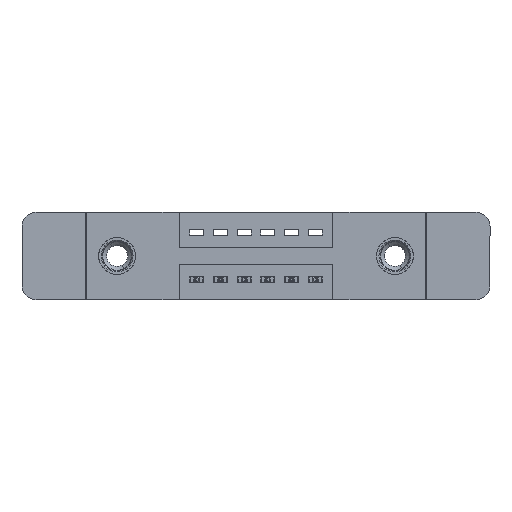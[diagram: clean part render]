
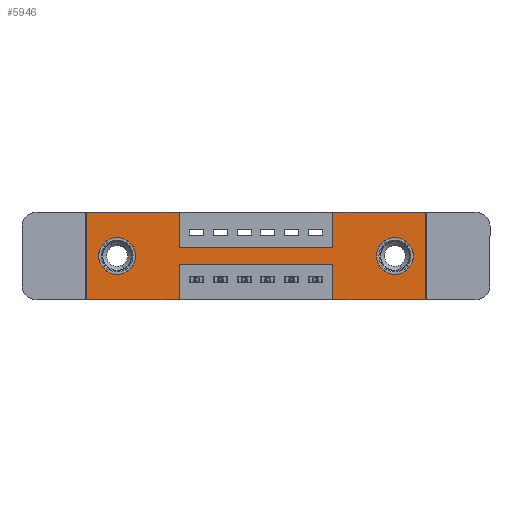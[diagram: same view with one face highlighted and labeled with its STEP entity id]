
A CAD part, front view. The second image highlights one B-rep face of the part: STEP entity #5946.
In plain terms, the highlighted planar face has unit normal (0, -1, 0).
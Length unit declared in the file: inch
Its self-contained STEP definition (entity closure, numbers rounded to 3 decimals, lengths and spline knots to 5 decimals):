
#244 = LINE ( 'NONE', #13794, #6252 ) ;
#265 = CIRCLE ( 'NONE', #1947, 0.078 ) ;
#278 = DIRECTION ( 'NONE',  ( 0., 0., -1. ) ) ;
#378 = DIRECTION ( 'NONE',  ( 0., 0., 1. ) ) ;
#475 = DIRECTION ( 'NONE',  ( -1., 0., 0. ) ) ;
#531 = VERTEX_POINT ( 'NONE', #13486 ) ;
#538 = VECTOR ( 'NONE', #7773, 39.37008 ) ;
#620 = CARTESIAN_POINT ( 'NONE',  ( 1.435, 0., -0.37 ) ) ;
#1287 = CIRCLE ( 'NONE', #2014, 0.078 ) ;
#1378 = EDGE_CURVE ( 'NONE', #5949, #7877, #12504, .T. ) ;
#1595 = VERTEX_POINT ( 'NONE', #13214 ) ;
#1741 = VECTOR ( 'NONE', #378, 39.37008 ) ;
#1817 = CARTESIAN_POINT ( 'NONE',  ( 0.3925, 0., -0.37 ) ) ;
#1819 = CARTESIAN_POINT ( 'NONE',  ( 0.3925, 0., -0.22 ) ) ;
#1947 = AXIS2_PLACEMENT_3D ( 'NONE', #5736, #12311, #6732 ) ;
#2014 = AXIS2_PLACEMENT_3D ( 'NONE', #12330, #12384, #6898 ) ;
#2072 = FACE_OUTER_BOUND ( 'NONE', #3925, .T. ) ;
#2209 = LINE ( 'NONE', #10895, #4870 ) ;
#2354 = VECTOR ( 'NONE', #8885, 39.37008 ) ;
#2723 = CARTESIAN_POINT ( 'NONE',  ( 1.0425, 0., 0. ) ) ;
#3039 = LINE ( 'NONE', #3862, #11682 ) ;
#3055 = CARTESIAN_POINT ( 'NONE',  ( 1.435, 0., 0. ) ) ;
#3166 = DIRECTION ( 'NONE',  ( 0., 0., -1. ) ) ;
#3187 = ORIENTED_EDGE ( 'NONE', *, *, #11785, .F. ) ;
#3298 = ORIENTED_EDGE ( 'NONE', *, *, #3936, .T. ) ;
#3303 = EDGE_CURVE ( 'NONE', #11059, #5215, #2209, .T. ) ;
#3304 = CARTESIAN_POINT ( 'NONE',  ( 1.0425, 0., -0.37 ) ) ;
#3393 = EDGE_CURVE ( 'NONE', #8481, #11059, #3789, .T. ) ;
#3515 = ORIENTED_EDGE ( 'NONE', *, *, #5880, .F. ) ;
#3595 = ORIENTED_EDGE ( 'NONE', *, *, #4989, .F. ) ;
#3655 = LINE ( 'NONE', #1819, #14251 ) ;
#3694 = DIRECTION ( 'NONE',  ( 0., 0., 1. ) ) ;
#3729 = LINE ( 'NONE', #3304, #538 ) ;
#3732 = CARTESIAN_POINT ( 'NONE',  ( 0., 0., 0. ) ) ;
#3789 = LINE ( 'NONE', #10486, #4155 ) ;
#3862 = CARTESIAN_POINT ( 'NONE',  ( 0., 0., 0. ) ) ;
#3925 = EDGE_LOOP ( 'NONE', ( #3595, #3515, #12734, #8670, #6734, #3187, #5157, #13919, #9355, #14100, #12618, #5961 ) ) ;
#3936 = EDGE_CURVE ( 'NONE', #531, #1595, #1287, .T. ) ;
#4110 = CARTESIAN_POINT ( 'NONE',  ( 1.0425, 0., -0.37 ) ) ;
#4155 = VECTOR ( 'NONE', #278, 39.37008 ) ;
#4364 = FACE_BOUND ( 'NONE', #7236, .T. ) ;
#4395 = CARTESIAN_POINT ( 'NONE',  ( 0., 0., -0.37 ) ) ;
#4492 = VECTOR ( 'NONE', #12124, 39.37008 ) ;
#4704 = EDGE_CURVE ( 'NONE', #14498, #14072, #244, .T. ) ;
#4748 = LINE ( 'NONE', #3732, #1741 ) ;
#4870 = VECTOR ( 'NONE', #12179, 39.37008 ) ;
#4989 = EDGE_CURVE ( 'NONE', #8682, #8084, #9417, .T. ) ;
#5077 = FACE_BOUND ( 'NONE', #5146, .T. ) ;
#5146 = EDGE_LOOP ( 'NONE', ( #13066, #9958 ) ) ;
#5157 = ORIENTED_EDGE ( 'NONE', *, *, #9910, .F. ) ;
#5215 = VERTEX_POINT ( 'NONE', #8140 ) ;
#5351 = CARTESIAN_POINT ( 'NONE',  ( 0.3925, 0., -0.37 ) ) ;
#5736 = CARTESIAN_POINT ( 'NONE',  ( 1.305, 0., -0.185 ) ) ;
#5878 = CARTESIAN_POINT ( 'NONE',  ( 1.0425, 0., 0. ) ) ;
#5880 = EDGE_CURVE ( 'NONE', #12254, #8682, #3655, .T. ) ;
#5946 = ADVANCED_FACE ( 'NONE', ( #5077, #4364, #2072 ), #7278, .T. ) ;
#5949 = VERTEX_POINT ( 'NONE', #8812 ) ;
#5961 = ORIENTED_EDGE ( 'NONE', *, *, #9845, .F. ) ;
#6208 = VECTOR ( 'NONE', #8326, 39.37008 ) ;
#6252 = VECTOR ( 'NONE', #8192, 39.37008 ) ;
#6527 = CARTESIAN_POINT ( 'NONE',  ( 1.0425, 0., -0.22 ) ) ;
#6732 = DIRECTION ( 'NONE',  ( 0., 0., -1. ) ) ;
#6734 = ORIENTED_EDGE ( 'NONE', *, *, #7230, .F. ) ;
#6753 = VERTEX_POINT ( 'NONE', #14349 ) ;
#6898 = DIRECTION ( 'NONE',  ( 0., 0., 1. ) ) ;
#6901 = EDGE_CURVE ( 'NONE', #7877, #5949, #265, .T. ) ;
#7230 = EDGE_CURVE ( 'NONE', #6753, #14498, #11904, .T. ) ;
#7236 = EDGE_LOOP ( 'NONE', ( #3298, #9581 ) ) ;
#7278 = PLANE ( 'NONE',  #9398 ) ;
#7397 = DIRECTION ( 'NONE',  ( 0., 1., 0. ) ) ;
#7773 = DIRECTION ( 'NONE',  ( 0., 0., 1. ) ) ;
#7777 = LINE ( 'NONE', #9518, #6208 ) ;
#7877 = VERTEX_POINT ( 'NONE', #10804 ) ;
#8084 = VERTEX_POINT ( 'NONE', #1817 ) ;
#8132 = VECTOR ( 'NONE', #10605, 39.37008 ) ;
#8140 = CARTESIAN_POINT ( 'NONE',  ( 1.0425, 0., -0.15 ) ) ;
#8192 = DIRECTION ( 'NONE',  ( -1., 0., 0. ) ) ;
#8256 = LINE ( 'NONE', #12017, #10922 ) ;
#8326 = DIRECTION ( 'NONE',  ( -1., 0., 0. ) ) ;
#8481 = VERTEX_POINT ( 'NONE', #8691 ) ;
#8543 = VERTEX_POINT ( 'NONE', #9862 ) ;
#8610 = CARTESIAN_POINT ( 'NONE',  ( 0., 0., -0.37 ) ) ;
#8663 = DIRECTION ( 'NONE',  ( 0., 0., -1. ) ) ;
#8670 = ORIENTED_EDGE ( 'NONE', *, *, #4704, .F. ) ;
#8682 = VERTEX_POINT ( 'NONE', #10302 ) ;
#8691 = CARTESIAN_POINT ( 'NONE',  ( 0.3925, 0., 0. ) ) ;
#8812 = CARTESIAN_POINT ( 'NONE',  ( 1.305, 0., -0.263 ) ) ;
#8885 = DIRECTION ( 'NONE',  ( 0., 0., -1. ) ) ;
#9355 = ORIENTED_EDGE ( 'NONE', *, *, #3393, .F. ) ;
#9398 = AXIS2_PLACEMENT_3D ( 'NONE', #8610, #12112, #8663 ) ;
#9417 = LINE ( 'NONE', #5351, #2354 ) ;
#9518 = CARTESIAN_POINT ( 'NONE',  ( 0., 0., -0.37 ) ) ;
#9581 = ORIENTED_EDGE ( 'NONE', *, *, #14347, .T. ) ;
#9617 = VERTEX_POINT ( 'NONE', #5878 ) ;
#9845 = EDGE_CURVE ( 'NONE', #8084, #11136, #7777, .T. ) ;
#9862 = CARTESIAN_POINT ( 'NONE',  ( 0., 0., 0. ) ) ;
#9910 = EDGE_CURVE ( 'NONE', #5215, #9617, #13995, .T. ) ;
#9947 = EDGE_CURVE ( 'NONE', #8543, #8481, #3039, .T. ) ;
#9958 = ORIENTED_EDGE ( 'NONE', *, *, #1378, .T. ) ;
#10144 = EDGE_CURVE ( 'NONE', #14072, #12254, #3729, .T. ) ;
#10236 = DIRECTION ( 'NONE',  ( 0., 1., 0. ) ) ;
#10285 = CARTESIAN_POINT ( 'NONE',  ( 0.13, 0., -0.185 ) ) ;
#10302 = CARTESIAN_POINT ( 'NONE',  ( 0.3925, 0., -0.22 ) ) ;
#10486 = CARTESIAN_POINT ( 'NONE',  ( 0.3925, 0., 0. ) ) ;
#10605 = DIRECTION ( 'NONE',  ( 0., 0., 1. ) ) ;
#10804 = CARTESIAN_POINT ( 'NONE',  ( 1.305, 0., -0.107 ) ) ;
#10861 = CARTESIAN_POINT ( 'NONE',  ( 0.3925, 0., -0.15 ) ) ;
#10895 = CARTESIAN_POINT ( 'NONE',  ( 0.3925, 0., -0.15 ) ) ;
#10922 = VECTOR ( 'NONE', #13175, 39.37008 ) ;
#10983 = AXIS2_PLACEMENT_3D ( 'NONE', #12933, #7397, #3166 ) ;
#11059 = VERTEX_POINT ( 'NONE', #10861 ) ;
#11114 = CIRCLE ( 'NONE', #13068, 0.078 ) ;
#11136 = VERTEX_POINT ( 'NONE', #4395 ) ;
#11682 = VECTOR ( 'NONE', #11741, 39.37008 ) ;
#11741 = DIRECTION ( 'NONE',  ( 1., 0., 0. ) ) ;
#11785 = EDGE_CURVE ( 'NONE', #9617, #6753, #8256, .T. ) ;
#11904 = LINE ( 'NONE', #3055, #4492 ) ;
#12017 = CARTESIAN_POINT ( 'NONE',  ( 0., 0., 0. ) ) ;
#12041 = EDGE_CURVE ( 'NONE', #11136, #8543, #4748, .T. ) ;
#12112 = DIRECTION ( 'NONE',  ( 0., -1., 0. ) ) ;
#12124 = DIRECTION ( 'NONE',  ( 0., 0., -1. ) ) ;
#12179 = DIRECTION ( 'NONE',  ( 1., 0., 0. ) ) ;
#12254 = VERTEX_POINT ( 'NONE', #6527 ) ;
#12311 = DIRECTION ( 'NONE',  ( 0., 1., 0. ) ) ;
#12330 = CARTESIAN_POINT ( 'NONE',  ( 0.13, 0., -0.185 ) ) ;
#12384 = DIRECTION ( 'NONE',  ( 0., 1., 0. ) ) ;
#12504 = CIRCLE ( 'NONE', #10983, 0.078 ) ;
#12618 = ORIENTED_EDGE ( 'NONE', *, *, #12041, .F. ) ;
#12734 = ORIENTED_EDGE ( 'NONE', *, *, #10144, .F. ) ;
#12933 = CARTESIAN_POINT ( 'NONE',  ( 1.305, 0., -0.185 ) ) ;
#13066 = ORIENTED_EDGE ( 'NONE', *, *, #6901, .T. ) ;
#13068 = AXIS2_PLACEMENT_3D ( 'NONE', #10285, #10236, #3694 ) ;
#13175 = DIRECTION ( 'NONE',  ( 1., 0., 0. ) ) ;
#13214 = CARTESIAN_POINT ( 'NONE',  ( 0.13, 0., -0.263 ) ) ;
#13486 = CARTESIAN_POINT ( 'NONE',  ( 0.13, 0., -0.107 ) ) ;
#13794 = CARTESIAN_POINT ( 'NONE',  ( 0., 0., -0.37 ) ) ;
#13919 = ORIENTED_EDGE ( 'NONE', *, *, #3303, .F. ) ;
#13995 = LINE ( 'NONE', #2723, #8132 ) ;
#14072 = VERTEX_POINT ( 'NONE', #4110 ) ;
#14100 = ORIENTED_EDGE ( 'NONE', *, *, #9947, .F. ) ;
#14251 = VECTOR ( 'NONE', #475, 39.37008 ) ;
#14347 = EDGE_CURVE ( 'NONE', #1595, #531, #11114, .T. ) ;
#14349 = CARTESIAN_POINT ( 'NONE',  ( 1.435, 0., 0. ) ) ;
#14498 = VERTEX_POINT ( 'NONE', #620 ) ;
